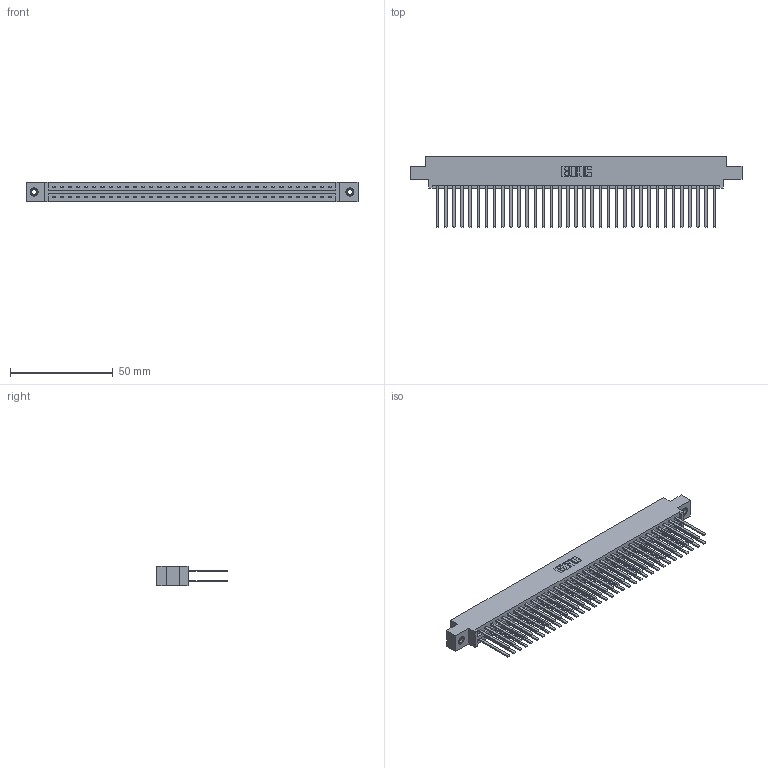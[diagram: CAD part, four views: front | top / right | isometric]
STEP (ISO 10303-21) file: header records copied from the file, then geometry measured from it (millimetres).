
FILE_DESCRIPTION (( 'STEP AP203' ), '1' );
FILE_NAME ('337-070-544-807.STEP', '2019-10-15T11:04:50', ( '' ), ( '' ), 'SwSTEP 2.0', 'SolidWorks 2016', '' );
FILE_SCHEMA (( 'CONFIG_CONTROL_DESIGN' ));
Length unit declared in the file: inch
Products named in the file (4): 337-070-544-807; 337 Part_0.170 Offset - 0.156 Dia-TI; 345-292-001_345-293-144; 345-250-001_345-250-005-103
Assembly tree (73 placements, depth 2):
  337-070-544-807
    337 Part_0.170 Offset - 0.156 Dia-TI
    345-292-001_345-293-144  x70
    345-250-001_345-250-005-103  x2
Bounding box: 161.7 x 34.3 x 9.4 mm (x, y, z)
Volume: 17797.9 mm3; surface area: 23401.9 mm2
Topology: 73 solids, 73 shells, 3538 faces, 10469 edges, 6878 vertices
Faces by surface type: plane 2486, cylinder 1036, cone 12, torus 4
Entity records: 29176 total; most frequent: CARTESIAN_POINT 4901, ORIENTED_EDGE 4830, DIRECTION 4209, EDGE_CURVE 2415, VECTOR 2271, LINE 2271, VERTEX_POINT 1604, AXIS2_PLACEMENT_3D 969
